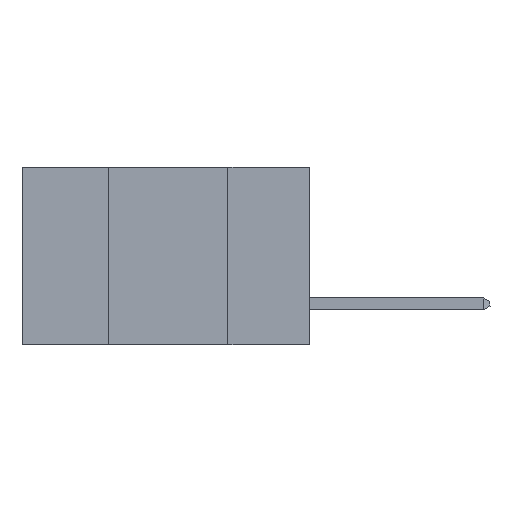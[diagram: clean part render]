
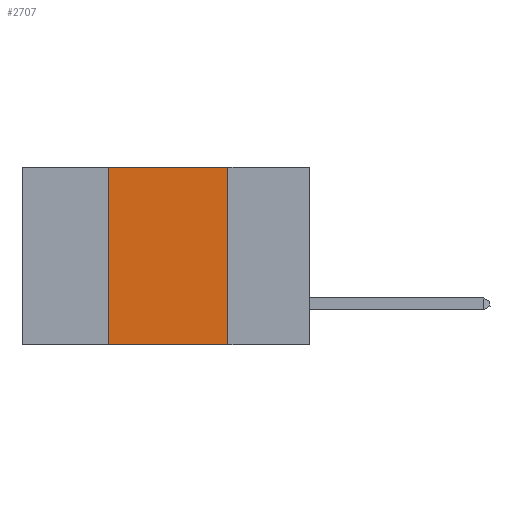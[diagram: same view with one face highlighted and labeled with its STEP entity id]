
A CAD part, left-side view. The second image highlights one B-rep face of the part: STEP entity #2707.
In plain terms, the highlighted planar face has unit normal (-1, 0, 0).
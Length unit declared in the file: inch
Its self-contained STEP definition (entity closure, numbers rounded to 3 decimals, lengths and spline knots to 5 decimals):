
#91 = LINE ( 'NONE', #8536, #3740 ) ;
#189 = CARTESIAN_POINT ( 'NONE',  ( 0., 0.17, -0.37 ) ) ;
#224 = ORIENTED_EDGE ( 'NONE', *, *, #8843, .F. ) ;
#545 = PLANE ( 'NONE',  #746 ) ;
#746 = AXIS2_PLACEMENT_3D ( 'NONE', #4023, #6127, #6061 ) ;
#979 = DIRECTION ( 'NONE',  ( 0., 0., 1. ) ) ;
#1314 = ORIENTED_EDGE ( 'NONE', *, *, #5310, .F. ) ;
#1468 = EDGE_CURVE ( 'NONE', #2390, #6760, #91, .T. ) ;
#1968 = EDGE_LOOP ( 'NONE', ( #3453, #224, #1314, #8353 ) ) ;
#2183 = VECTOR ( 'NONE', #3691, 39.37008 ) ;
#2390 = VERTEX_POINT ( 'NONE', #6075 ) ;
#2633 = CARTESIAN_POINT ( 'NONE',  ( 0., 0.6, -0.37 ) ) ;
#2707 = ADVANCED_FACE ( 'NONE', ( #2781 ), #545, .F. ) ;
#2781 = FACE_OUTER_BOUND ( 'NONE', #1968, .T. ) ;
#2906 = VERTEX_POINT ( 'NONE', #7830 ) ;
#2975 = VECTOR ( 'NONE', #7451, 39.37008 ) ;
#2981 = CARTESIAN_POINT ( 'NONE',  ( 0., 0.42, 0. ) ) ;
#3096 = VERTEX_POINT ( 'NONE', #8618 ) ;
#3345 = EDGE_CURVE ( 'NONE', #2906, #6760, #4801, .T. ) ;
#3453 = ORIENTED_EDGE ( 'NONE', *, *, #1468, .F. ) ;
#3691 = DIRECTION ( 'NONE',  ( 0., -1., 0. ) ) ;
#3740 = VECTOR ( 'NONE', #4411, 39.37008 ) ;
#4023 = CARTESIAN_POINT ( 'NONE',  ( 0., 0.6, 0. ) ) ;
#4411 = DIRECTION ( 'NONE',  ( 0., 0., -1. ) ) ;
#4553 = VECTOR ( 'NONE', #979, 39.37008 ) ;
#4801 = LINE ( 'NONE', #2633, #2975 ) ;
#5089 = LINE ( 'NONE', #2981, #4553 ) ;
#5094 = LINE ( 'NONE', #7264, #2183 ) ;
#5310 = EDGE_CURVE ( 'NONE', #2906, #3096, #5089, .T. ) ;
#6061 = DIRECTION ( 'NONE',  ( 0., 0., -1. ) ) ;
#6075 = CARTESIAN_POINT ( 'NONE',  ( 0., 0.17, 0. ) ) ;
#6127 = DIRECTION ( 'NONE',  ( 1., 0., 0. ) ) ;
#6760 = VERTEX_POINT ( 'NONE', #189 ) ;
#7264 = CARTESIAN_POINT ( 'NONE',  ( 0., 0.6, 0. ) ) ;
#7451 = DIRECTION ( 'NONE',  ( 0., -1., 0. ) ) ;
#7830 = CARTESIAN_POINT ( 'NONE',  ( 0., 0.42, -0.37 ) ) ;
#8353 = ORIENTED_EDGE ( 'NONE', *, *, #3345, .T. ) ;
#8536 = CARTESIAN_POINT ( 'NONE',  ( 0., 0.17, 0. ) ) ;
#8618 = CARTESIAN_POINT ( 'NONE',  ( 0., 0.42, 0. ) ) ;
#8843 = EDGE_CURVE ( 'NONE', #3096, #2390, #5094, .T. ) ;
